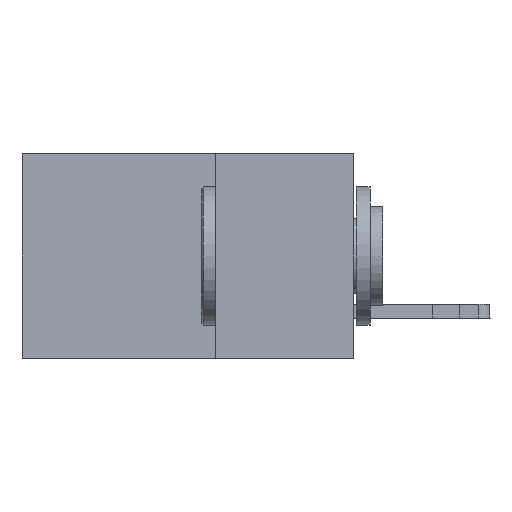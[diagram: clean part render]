
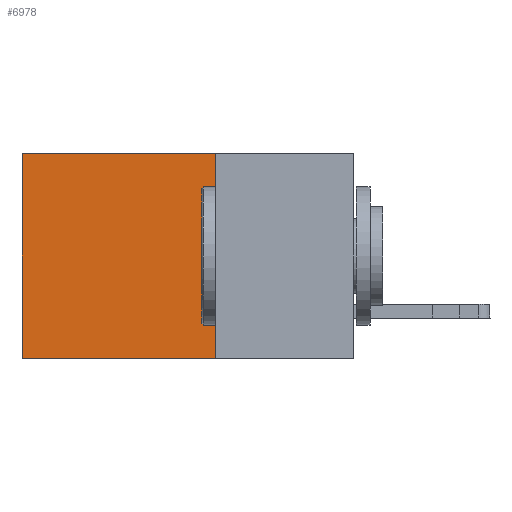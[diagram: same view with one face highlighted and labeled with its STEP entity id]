
A CAD part, left-side view. The second image highlights one B-rep face of the part: STEP entity #6978.
In plain terms, the highlighted planar face has unit normal (-1, 0, 0).
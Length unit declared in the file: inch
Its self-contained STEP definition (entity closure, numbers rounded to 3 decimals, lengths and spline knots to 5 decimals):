
#2707 = ORIENTED_EDGE ( 'NONE', *, *, #23645, .F. ) ;
#3414 = EDGE_CURVE ( 'NONE', #18614, #9736, #4331, .T. ) ;
#3467 = DIRECTION ( 'NONE',  ( 0., 0., -1. ) ) ;
#4063 = VECTOR ( 'NONE', #6955, 39.37008 ) ;
#4096 = VECTOR ( 'NONE', #14852, 39.37008 ) ;
#4331 = LINE ( 'NONE', #17557, #4096 ) ;
#5067 = ORIENTED_EDGE ( 'NONE', *, *, #15160, .T. ) ;
#5907 = VECTOR ( 'NONE', #14945, 39.37008 ) ;
#6955 = DIRECTION ( 'NONE',  ( 0., 1., 0. ) ) ;
#6978 = ADVANCED_FACE ( 'NONE', ( #24914 ), #26747, .F. ) ;
#8456 = ORIENTED_EDGE ( 'NONE', *, *, #3414, .T. ) ;
#9736 = VERTEX_POINT ( 'NONE', #10531 ) ;
#9890 = ORIENTED_EDGE ( 'NONE', *, *, #19087, .F. ) ;
#10531 = CARTESIAN_POINT ( 'NONE',  ( 0.2875, 0.6, 0. ) ) ;
#11286 = VERTEX_POINT ( 'NONE', #16128 ) ;
#12742 = VERTEX_POINT ( 'NONE', #15025 ) ;
#12985 = EDGE_LOOP ( 'NONE', ( #5067, #9890, #2707, #8456 ) ) ;
#13669 = DIRECTION ( 'NONE',  ( 0., 0., -1. ) ) ;
#14584 = AXIS2_PLACEMENT_3D ( 'NONE', #27030, #26883, #3467 ) ;
#14852 = DIRECTION ( 'NONE',  ( 0., 1., 0. ) ) ;
#14945 = DIRECTION ( 'NONE',  ( 0., 0., -1. ) ) ;
#15025 = CARTESIAN_POINT ( 'NONE',  ( 0.2875, 0.25, -0.37 ) ) ;
#15160 = EDGE_CURVE ( 'NONE', #9736, #11286, #24835, .T. ) ;
#15783 = CARTESIAN_POINT ( 'NONE',  ( 0.2875, 0.6, 0. ) ) ;
#16128 = CARTESIAN_POINT ( 'NONE',  ( 0.2875, 0.6, -0.37 ) ) ;
#16770 = CARTESIAN_POINT ( 'NONE',  ( 0.2875, 0.25, 0. ) ) ;
#17442 = VECTOR ( 'NONE', #13669, 39.37008 ) ;
#17547 = CARTESIAN_POINT ( 'NONE',  ( 0.2875, 0.25, 0. ) ) ;
#17557 = CARTESIAN_POINT ( 'NONE',  ( 0.2875, 0.25, 0. ) ) ;
#18614 = VERTEX_POINT ( 'NONE', #17547 ) ;
#19087 = EDGE_CURVE ( 'NONE', #12742, #11286, #23898, .T. ) ;
#23645 = EDGE_CURVE ( 'NONE', #18614, #12742, #25545, .T. ) ;
#23898 = LINE ( 'NONE', #26300, #4063 ) ;
#24835 = LINE ( 'NONE', #15783, #17442 ) ;
#24914 = FACE_OUTER_BOUND ( 'NONE', #12985, .T. ) ;
#25545 = LINE ( 'NONE', #16770, #5907 ) ;
#26300 = CARTESIAN_POINT ( 'NONE',  ( 0.2875, 0.25, -0.37 ) ) ;
#26747 = PLANE ( 'NONE',  #14584 ) ;
#26883 = DIRECTION ( 'NONE',  ( 1., 0., 0. ) ) ;
#27030 = CARTESIAN_POINT ( 'NONE',  ( 0.2875, 0.25, 0. ) ) ;
